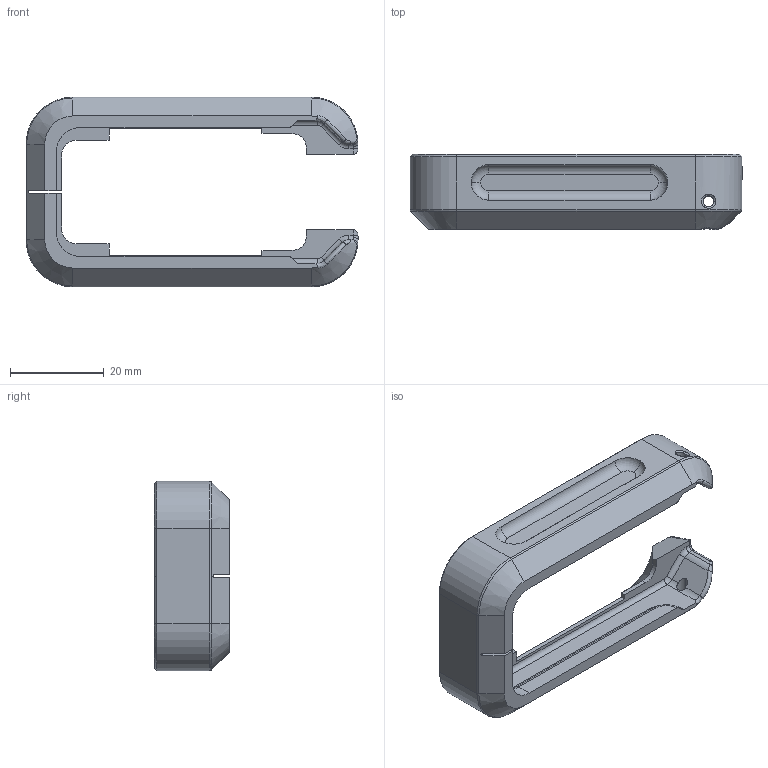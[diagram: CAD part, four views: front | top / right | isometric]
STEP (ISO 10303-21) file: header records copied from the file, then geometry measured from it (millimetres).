
FILE_DESCRIPTION (( 'STEP AP214' ), '1' );
FILE_NAME ('Flared_Magwell_V2.STEP', '2025-07-07T03:53:05', ( '' ), ( '' ), 'SwSTEP 2.0', 'SolidWorks 2020', '' );
FILE_SCHEMA (( 'AUTOMOTIVE_DESIGN' ));
Length unit declared in the file: millimetre
Products named in the file (1): Flared_Magwell_V2
Bounding box: 70.77 x 16.02 x 40.4 mm (x, y, z)
Volume: 12322.5 mm3; surface area: 7640.8 mm2
Topology: 1 solids, 1 shells, 182 faces, 450 edges, 270 vertices
Faces by surface type: plane 67, cylinder 51, torus 28, bspline 20, cone 16
Entity records: 8230 total; most frequent: CARTESIAN_POINT 4015, ORIENTED_EDGE 900, DIRECTION 858, EDGE_CURVE 450, AXIS2_PLACEMENT_3D 317, VERTEX_POINT 270, VECTOR 224, LINE 224
